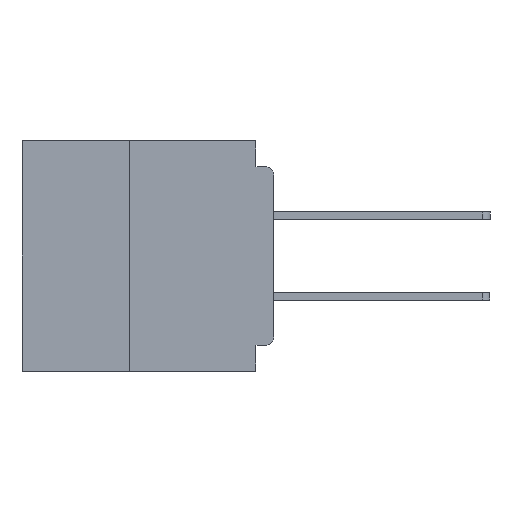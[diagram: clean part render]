
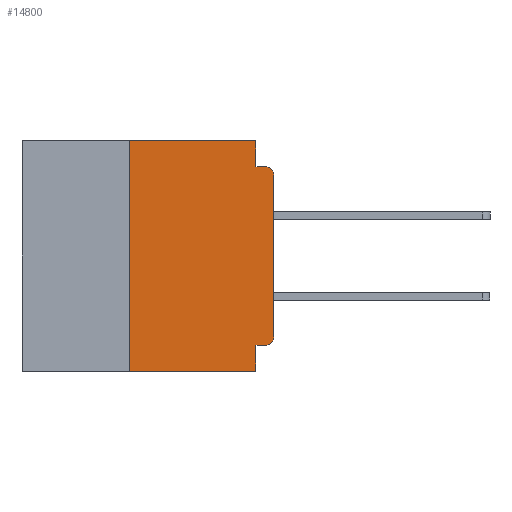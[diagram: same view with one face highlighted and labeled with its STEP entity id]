
A CAD part, left-side view. The second image highlights one B-rep face of the part: STEP entity #14800.
In plain terms, the highlighted planar face has unit normal (-1, 0, 0).
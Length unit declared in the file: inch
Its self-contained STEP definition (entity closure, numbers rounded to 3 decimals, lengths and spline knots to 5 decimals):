
#138 = DIRECTION ( 'NONE',  ( 0., 0., -1. ) ) ;
#2322 = CARTESIAN_POINT ( 'NONE',  ( 0., 0.031, 0. ) ) ;
#3007 = DIRECTION ( 'NONE',  ( 0., 0., 1. ) ) ;
#3013 = VERTEX_POINT ( 'NONE', #5603 ) ;
#3318 = VECTOR ( 'NONE', #15288, 39.37008 ) ;
#5560 = CARTESIAN_POINT ( 'NONE',  ( 0., 0.015, -0.045 ) ) ;
#5603 = CARTESIAN_POINT ( 'NONE',  ( 0., 0., -0.06 ) ) ;
#6143 = CARTESIAN_POINT ( 'NONE',  ( 0., 0.25, -0.4 ) ) ;
#7023 = ORIENTED_EDGE ( 'NONE', *, *, #17376, .F. ) ;
#7414 = CARTESIAN_POINT ( 'NONE',  ( 0., 0.031, 0. ) ) ;
#7419 = EDGE_CURVE ( 'NONE', #20685, #29228, #19153, .T. ) ;
#7528 = VERTEX_POINT ( 'NONE', #33252 ) ;
#8278 = VECTOR ( 'NONE', #138, 39.37008 ) ;
#8508 = VECTOR ( 'NONE', #13427, 39.37008 ) ;
#8998 = AXIS2_PLACEMENT_3D ( 'NONE', #9509, #12725, #34898 ) ;
#9448 = DIRECTION ( 'NONE',  ( -1., 0., 0. ) ) ;
#9509 = CARTESIAN_POINT ( 'NONE',  ( 0., 0.437, 0. ) ) ;
#9649 = EDGE_CURVE ( 'NONE', #20685, #18213, #17965, .T. ) ;
#9690 = VERTEX_POINT ( 'NONE', #7414 ) ;
#11307 = LINE ( 'NONE', #28503, #26253 ) ;
#11732 = ORIENTED_EDGE ( 'NONE', *, *, #26882, .F. ) ;
#11836 = LINE ( 'NONE', #37436, #3318 ) ;
#12314 = EDGE_CURVE ( 'NONE', #29228, #3013, #25775, .T. ) ;
#12725 = DIRECTION ( 'NONE',  ( 1., 0., 0. ) ) ;
#12923 = DIRECTION ( 'NONE',  ( 0., -1., 0. ) ) ;
#13331 = VECTOR ( 'NONE', #12923, 39.37008 ) ;
#13427 = DIRECTION ( 'NONE',  ( 0., 1., 0. ) ) ;
#13716 = DIRECTION ( 'NONE',  ( -1., 0., 0. ) ) ;
#14800 = ADVANCED_FACE ( 'NONE', ( #27530 ), #28547, .F. ) ;
#15288 = DIRECTION ( 'NONE',  ( 0., -1., 0. ) ) ;
#16389 = AXIS2_PLACEMENT_3D ( 'NONE', #32725, #13716, #35895 ) ;
#16745 = LINE ( 'NONE', #34905, #8278 ) ;
#16842 = LINE ( 'NONE', #2322, #40080 ) ;
#17026 = ORIENTED_EDGE ( 'NONE', *, *, #12314, .T. ) ;
#17204 = VECTOR ( 'NONE', #36297, 39.37008 ) ;
#17312 = VECTOR ( 'NONE', #40363, 39.37008 ) ;
#17376 = EDGE_CURVE ( 'NONE', #9690, #39496, #16842, .T. ) ;
#17965 = LINE ( 'NONE', #32585, #8508 ) ;
#18189 = LINE ( 'NONE', #32978, #17204 ) ;
#18213 = VERTEX_POINT ( 'NONE', #22768 ) ;
#19153 = CIRCLE ( 'NONE', #16389, 0.015 ) ;
#20286 = ORIENTED_EDGE ( 'NONE', *, *, #22070, .F. ) ;
#20480 = ORIENTED_EDGE ( 'NONE', *, *, #7419, .T. ) ;
#20685 = VERTEX_POINT ( 'NONE', #29509 ) ;
#22070 = EDGE_CURVE ( 'NONE', #39496, #29573, #18189, .T. ) ;
#22504 = ORIENTED_EDGE ( 'NONE', *, *, #27490, .F. ) ;
#22681 = CARTESIAN_POINT ( 'NONE',  ( 0., 0.031, -0.045 ) ) ;
#22768 = CARTESIAN_POINT ( 'NONE',  ( 0., 0.031, -0.355 ) ) ;
#22913 = CARTESIAN_POINT ( 'NONE',  ( 0., 0., -0.34 ) ) ;
#23226 = ORIENTED_EDGE ( 'NONE', *, *, #26704, .T. ) ;
#23370 = AXIS2_PLACEMENT_3D ( 'NONE', #28484, #9448, #31669 ) ;
#24378 = CARTESIAN_POINT ( 'NONE',  ( 0., 0., 0. ) ) ;
#25775 = LINE ( 'NONE', #24378, #17312 ) ;
#26253 = VECTOR ( 'NONE', #3007, 39.37008 ) ;
#26620 = CIRCLE ( 'NONE', #23370, 0.015 ) ;
#26704 = EDGE_CURVE ( 'NONE', #31466, #31794, #11836, .T. ) ;
#26882 = EDGE_CURVE ( 'NONE', #7528, #9690, #31213, .T. ) ;
#27490 = EDGE_CURVE ( 'NONE', #18213, #31794, #16745, .T. ) ;
#27530 = FACE_OUTER_BOUND ( 'NONE', #35771, .T. ) ;
#27605 = ORIENTED_EDGE ( 'NONE', *, *, #9649, .F. ) ;
#27666 = DIRECTION ( 'NONE',  ( 0., 0., -1. ) ) ;
#28484 = CARTESIAN_POINT ( 'NONE',  ( 0., 0.015, -0.06 ) ) ;
#28503 = CARTESIAN_POINT ( 'NONE',  ( 0., 0.25, -0.4 ) ) ;
#28513 = EDGE_CURVE ( 'NONE', #3013, #29573, #26620, .T. ) ;
#28547 = PLANE ( 'NONE',  #8998 ) ;
#29228 = VERTEX_POINT ( 'NONE', #22913 ) ;
#29509 = CARTESIAN_POINT ( 'NONE',  ( 0., 0.015, -0.355 ) ) ;
#29573 = VERTEX_POINT ( 'NONE', #5560 ) ;
#31213 = LINE ( 'NONE', #35092, #13331 ) ;
#31466 = VERTEX_POINT ( 'NONE', #6143 ) ;
#31669 = DIRECTION ( 'NONE',  ( 0., 0., -1. ) ) ;
#31794 = VERTEX_POINT ( 'NONE', #36533 ) ;
#32585 = CARTESIAN_POINT ( 'NONE',  ( 0., 0., -0.355 ) ) ;
#32725 = CARTESIAN_POINT ( 'NONE',  ( 0., 0.015, -0.34 ) ) ;
#32978 = CARTESIAN_POINT ( 'NONE',  ( 0., 0., -0.045 ) ) ;
#33252 = CARTESIAN_POINT ( 'NONE',  ( 0., 0.25, 0. ) ) ;
#34898 = DIRECTION ( 'NONE',  ( 0., 0., -1. ) ) ;
#34905 = CARTESIAN_POINT ( 'NONE',  ( 0., 0.031, -0.4 ) ) ;
#35092 = CARTESIAN_POINT ( 'NONE',  ( 0., 0.437, 0. ) ) ;
#35771 = EDGE_LOOP ( 'NONE', ( #17026, #40323, #20286, #7023, #11732, #38908, #23226, #22504, #27605, #20480 ) ) ;
#35895 = DIRECTION ( 'NONE',  ( 0., 0., -1. ) ) ;
#36297 = DIRECTION ( 'NONE',  ( 0., -1., 0. ) ) ;
#36533 = CARTESIAN_POINT ( 'NONE',  ( 0., 0.031, -0.4 ) ) ;
#37436 = CARTESIAN_POINT ( 'NONE',  ( 0., 0.437, -0.4 ) ) ;
#38908 = ORIENTED_EDGE ( 'NONE', *, *, #39379, .F. ) ;
#39379 = EDGE_CURVE ( 'NONE', #31466, #7528, #11307, .T. ) ;
#39496 = VERTEX_POINT ( 'NONE', #22681 ) ;
#40080 = VECTOR ( 'NONE', #27666, 39.37008 ) ;
#40323 = ORIENTED_EDGE ( 'NONE', *, *, #28513, .T. ) ;
#40363 = DIRECTION ( 'NONE',  ( 0., 0., 1. ) ) ;
